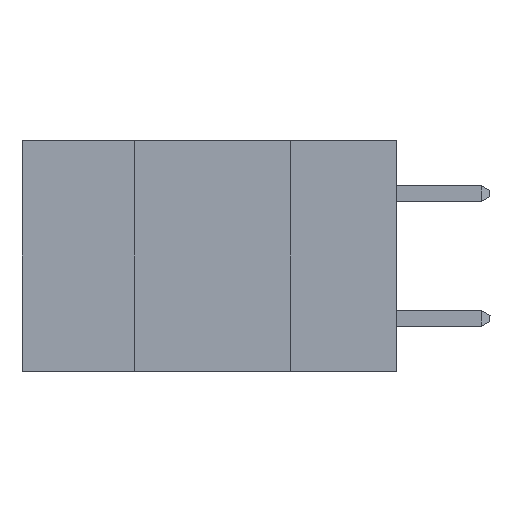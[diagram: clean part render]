
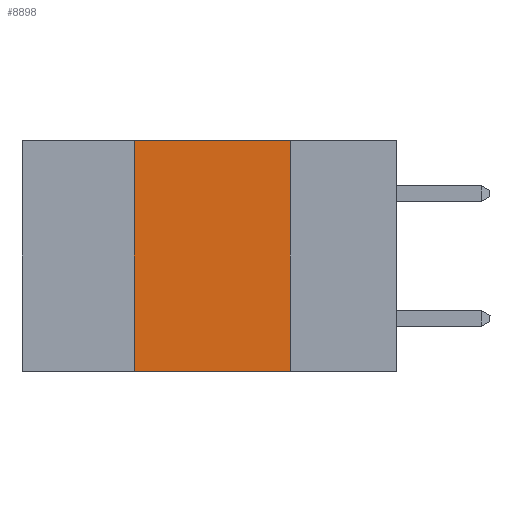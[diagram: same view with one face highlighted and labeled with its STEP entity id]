
A CAD part, left-side view. The second image highlights one B-rep face of the part: STEP entity #8898.
In plain terms, the highlighted planar face has unit normal (-1, 0, 0).
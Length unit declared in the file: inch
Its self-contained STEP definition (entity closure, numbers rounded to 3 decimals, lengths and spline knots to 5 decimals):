
#14 = LINE ( 'NONE', #919, #19109 ) ;
#919 = CARTESIAN_POINT ( 'NONE',  ( 0., 0.6, 0. ) ) ;
#1348 = ORIENTED_EDGE ( 'NONE', *, *, #10486, .F. ) ;
#2926 = EDGE_LOOP ( 'NONE', ( #7278, #9608, #1348, #12572 ) ) ;
#4057 = VERTEX_POINT ( 'NONE', #23253 ) ;
#4258 = PLANE ( 'NONE',  #5157 ) ;
#4606 = EDGE_CURVE ( 'NONE', #19860, #21132, #14, .T. ) ;
#5157 = AXIS2_PLACEMENT_3D ( 'NONE', #10455, #22914, #6591 ) ;
#6591 = DIRECTION ( 'NONE',  ( 0., 0., -1. ) ) ;
#6948 = CARTESIAN_POINT ( 'NONE',  ( 0., 0.17, 0. ) ) ;
#7056 = CARTESIAN_POINT ( 'NONE',  ( 0., 0.42, 0. ) ) ;
#7278 = ORIENTED_EDGE ( 'NONE', *, *, #15859, .F. ) ;
#8898 = ADVANCED_FACE ( 'NONE', ( #15275 ), #4258, .F. ) ;
#9608 = ORIENTED_EDGE ( 'NONE', *, *, #4606, .F. ) ;
#10455 = CARTESIAN_POINT ( 'NONE',  ( 0., 0.6, 0. ) ) ;
#10467 = DIRECTION ( 'NONE',  ( 0., 0., -1. ) ) ;
#10469 = LINE ( 'NONE', #16604, #17547 ) ;
#10486 = EDGE_CURVE ( 'NONE', #4057, #19860, #22677, .T. ) ;
#11757 = EDGE_CURVE ( 'NONE', #4057, #22234, #13887, .T. ) ;
#11825 = CARTESIAN_POINT ( 'NONE',  ( 0., 0.17, -0.37 ) ) ;
#12325 = VECTOR ( 'NONE', #23105, 39.37008 ) ;
#12572 = ORIENTED_EDGE ( 'NONE', *, *, #11757, .T. ) ;
#13188 = DIRECTION ( 'NONE',  ( 0., -1., 0. ) ) ;
#13751 = DIRECTION ( 'NONE',  ( 0., -1., 0. ) ) ;
#13887 = LINE ( 'NONE', #26169, #19063 ) ;
#15275 = FACE_OUTER_BOUND ( 'NONE', #2926, .T. ) ;
#15859 = EDGE_CURVE ( 'NONE', #21132, #22234, #10469, .T. ) ;
#16604 = CARTESIAN_POINT ( 'NONE',  ( 0., 0.17, 0. ) ) ;
#17547 = VECTOR ( 'NONE', #10467, 39.37008 ) ;
#18479 = CARTESIAN_POINT ( 'NONE',  ( 0., 0.42, 0. ) ) ;
#19063 = VECTOR ( 'NONE', #13751, 39.37008 ) ;
#19109 = VECTOR ( 'NONE', #13188, 39.37008 ) ;
#19860 = VERTEX_POINT ( 'NONE', #18479 ) ;
#21132 = VERTEX_POINT ( 'NONE', #6948 ) ;
#22234 = VERTEX_POINT ( 'NONE', #11825 ) ;
#22677 = LINE ( 'NONE', #7056, #12325 ) ;
#22914 = DIRECTION ( 'NONE',  ( 1., 0., 0. ) ) ;
#23105 = DIRECTION ( 'NONE',  ( 0., 0., 1. ) ) ;
#23253 = CARTESIAN_POINT ( 'NONE',  ( 0., 0.42, -0.37 ) ) ;
#26169 = CARTESIAN_POINT ( 'NONE',  ( 0., 0.6, -0.37 ) ) ;
